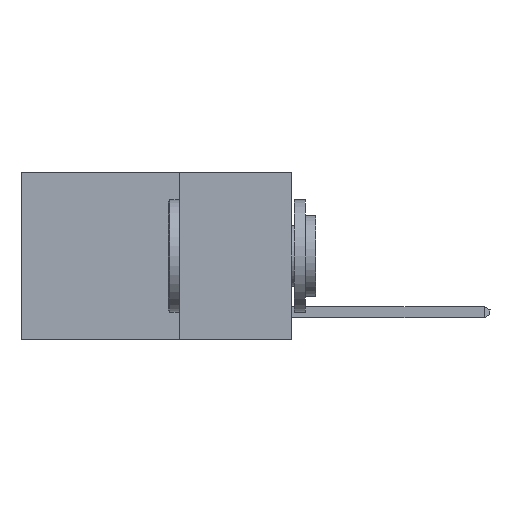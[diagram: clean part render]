
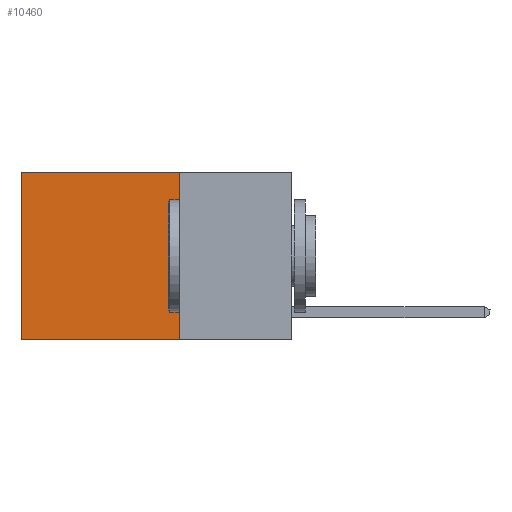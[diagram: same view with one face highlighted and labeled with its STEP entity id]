
A CAD part, left-side view. The second image highlights one B-rep face of the part: STEP entity #10460.
In plain terms, the highlighted planar face has unit normal (-1, 0, 0).
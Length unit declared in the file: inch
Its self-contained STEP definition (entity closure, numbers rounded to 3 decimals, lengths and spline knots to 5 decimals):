
#309 = LINE ( 'NONE', #8179, #5306 ) ;
#543 = EDGE_CURVE ( 'NONE', #22189, #13174, #5303, .T. ) ;
#1223 = DIRECTION ( 'NONE',  ( 0., 0., -1. ) ) ;
#1910 = ORIENTED_EDGE ( 'NONE', *, *, #23027, .F. ) ;
#3732 = VECTOR ( 'NONE', #9245, 39.37008 ) ;
#4561 = AXIS2_PLACEMENT_3D ( 'NONE', #5341, #20011, #7470 ) ;
#4992 = CARTESIAN_POINT ( 'NONE',  ( 0.2625, 0.25, 0. ) ) ;
#5303 = LINE ( 'NONE', #17860, #26943 ) ;
#5306 = VECTOR ( 'NONE', #24894, 39.37008 ) ;
#5341 = CARTESIAN_POINT ( 'NONE',  ( 0.2625, 0.25, 0. ) ) ;
#6538 = VERTEX_POINT ( 'NONE', #26372 ) ;
#7470 = DIRECTION ( 'NONE',  ( 0., 0., -1. ) ) ;
#8179 = CARTESIAN_POINT ( 'NONE',  ( 0.2625, 0.25, -0.37 ) ) ;
#9245 = DIRECTION ( 'NONE',  ( 0., 1., 0. ) ) ;
#9344 = LINE ( 'NONE', #4992, #3732 ) ;
#10460 = ADVANCED_FACE ( 'NONE', ( #13619 ), #13622, .F. ) ;
#11262 = CARTESIAN_POINT ( 'NONE',  ( 0.2625, 0.6, 0. ) ) ;
#11840 = ORIENTED_EDGE ( 'NONE', *, *, #13847, .F. ) ;
#13174 = VERTEX_POINT ( 'NONE', #20550 ) ;
#13280 = ORIENTED_EDGE ( 'NONE', *, *, #23544, .T. ) ;
#13619 = FACE_OUTER_BOUND ( 'NONE', #27161, .T. ) ;
#13622 = PLANE ( 'NONE',  #4561 ) ;
#13847 = EDGE_CURVE ( 'NONE', #26161, #13174, #309, .T. ) ;
#17860 = CARTESIAN_POINT ( 'NONE',  ( 0.2625, 0.6, 0. ) ) ;
#18068 = DIRECTION ( 'NONE',  ( 0., 0., -1. ) ) ;
#19377 = CARTESIAN_POINT ( 'NONE',  ( 0.2625, 0.25, -0.37 ) ) ;
#20011 = DIRECTION ( 'NONE',  ( 1., 0., 0. ) ) ;
#20550 = CARTESIAN_POINT ( 'NONE',  ( 0.2625, 0.6, -0.37 ) ) ;
#22189 = VERTEX_POINT ( 'NONE', #11262 ) ;
#22471 = VECTOR ( 'NONE', #1223, 39.37008 ) ;
#23027 = EDGE_CURVE ( 'NONE', #6538, #26161, #23130, .T. ) ;
#23130 = LINE ( 'NONE', #26375, #22471 ) ;
#23544 = EDGE_CURVE ( 'NONE', #6538, #22189, #9344, .T. ) ;
#24220 = ORIENTED_EDGE ( 'NONE', *, *, #543, .T. ) ;
#24894 = DIRECTION ( 'NONE',  ( 0., 1., 0. ) ) ;
#26161 = VERTEX_POINT ( 'NONE', #19377 ) ;
#26372 = CARTESIAN_POINT ( 'NONE',  ( 0.2625, 0.25, 0. ) ) ;
#26375 = CARTESIAN_POINT ( 'NONE',  ( 0.2625, 0.25, 0. ) ) ;
#26943 = VECTOR ( 'NONE', #18068, 39.37008 ) ;
#27161 = EDGE_LOOP ( 'NONE', ( #24220, #11840, #1910, #13280 ) ) ;
